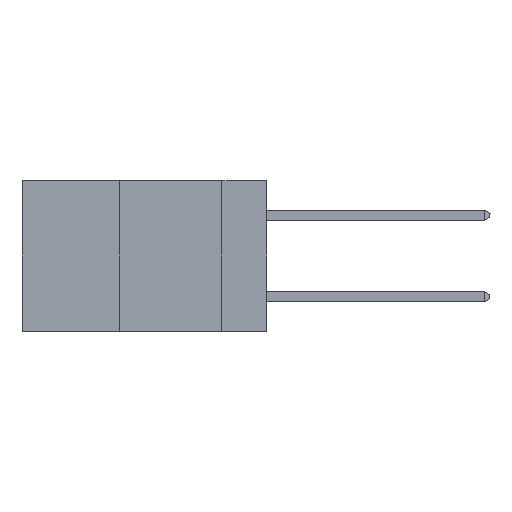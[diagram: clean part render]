
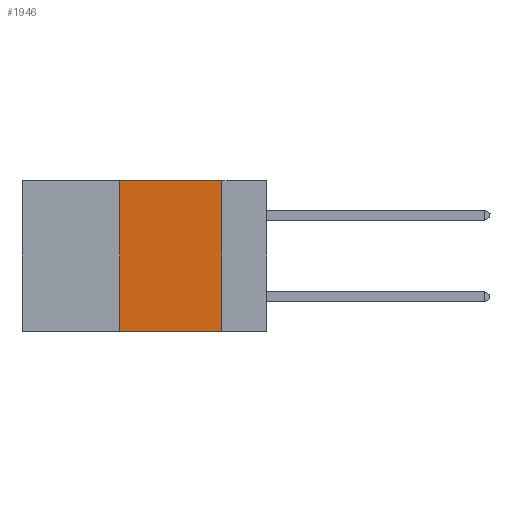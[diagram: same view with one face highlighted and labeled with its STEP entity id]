
A CAD part, left-side view. The second image highlights one B-rep face of the part: STEP entity #1946.
In plain terms, the highlighted planar face has unit normal (-1, 0, 0).
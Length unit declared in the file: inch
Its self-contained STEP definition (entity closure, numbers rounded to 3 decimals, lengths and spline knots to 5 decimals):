
#357 = VERTEX_POINT ( 'NONE', #3621 ) ;
#442 = EDGE_CURVE ( 'NONE', #10815, #970, #4486, .T. ) ;
#492 = VERTEX_POINT ( 'NONE', #4055 ) ;
#970 = VERTEX_POINT ( 'NONE', #9850 ) ;
#1120 = DIRECTION ( 'NONE',  ( 0., 0., -1. ) ) ;
#1946 = ADVANCED_FACE ( 'NONE', ( #9741 ), #7758, .F. ) ;
#2352 = CARTESIAN_POINT ( 'NONE',  ( 0., 0.6, 0. ) ) ;
#2518 = VECTOR ( 'NONE', #1120, 39.37008 ) ;
#2540 = EDGE_CURVE ( 'NONE', #492, #970, #5136, .T. ) ;
#3621 = CARTESIAN_POINT ( 'NONE',  ( 0., 0.36, 0. ) ) ;
#4055 = CARTESIAN_POINT ( 'NONE',  ( 0., 0.11, 0. ) ) ;
#4332 = CARTESIAN_POINT ( 'NONE',  ( 0., 0.11, 0. ) ) ;
#4486 = LINE ( 'NONE', #9675, #9241 ) ;
#5136 = LINE ( 'NONE', #4332, #2518 ) ;
#5379 = LINE ( 'NONE', #2352, #10107 ) ;
#5395 = DIRECTION ( 'NONE',  ( 0., 0., 1. ) ) ;
#5659 = EDGE_CURVE ( 'NONE', #357, #492, #5379, .T. ) ;
#5717 = CARTESIAN_POINT ( 'NONE',  ( 0., 0.36, -0.37 ) ) ;
#6304 = AXIS2_PLACEMENT_3D ( 'NONE', #7569, #7558, #7544 ) ;
#6856 = ORIENTED_EDGE ( 'NONE', *, *, #442, .T. ) ;
#7402 = ORIENTED_EDGE ( 'NONE', *, *, #5659, .F. ) ;
#7544 = DIRECTION ( 'NONE',  ( 0., 0., -1. ) ) ;
#7558 = DIRECTION ( 'NONE',  ( 1., 0., 0. ) ) ;
#7569 = CARTESIAN_POINT ( 'NONE',  ( 0., 0.6, 0. ) ) ;
#7758 = PLANE ( 'NONE',  #6304 ) ;
#8631 = EDGE_LOOP ( 'NONE', ( #10760, #7402, #9089, #6856 ) ) ;
#8907 = CARTESIAN_POINT ( 'NONE',  ( 0., 0.36, 0. ) ) ;
#9089 = ORIENTED_EDGE ( 'NONE', *, *, #11453, .F. ) ;
#9241 = VECTOR ( 'NONE', #9525, 39.37008 ) ;
#9308 = VECTOR ( 'NONE', #5395, 39.37008 ) ;
#9525 = DIRECTION ( 'NONE',  ( 0., -1., 0. ) ) ;
#9675 = CARTESIAN_POINT ( 'NONE',  ( 0., 0.6, -0.37 ) ) ;
#9741 = FACE_OUTER_BOUND ( 'NONE', #8631, .T. ) ;
#9850 = CARTESIAN_POINT ( 'NONE',  ( 0., 0.11, -0.37 ) ) ;
#10107 = VECTOR ( 'NONE', #10722, 39.37008 ) ;
#10722 = DIRECTION ( 'NONE',  ( 0., -1., 0. ) ) ;
#10760 = ORIENTED_EDGE ( 'NONE', *, *, #2540, .F. ) ;
#10815 = VERTEX_POINT ( 'NONE', #5717 ) ;
#11453 = EDGE_CURVE ( 'NONE', #10815, #357, #11717, .T. ) ;
#11717 = LINE ( 'NONE', #8907, #9308 ) ;
